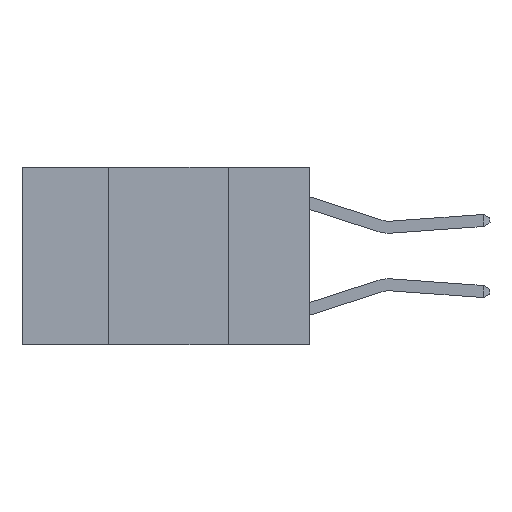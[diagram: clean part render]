
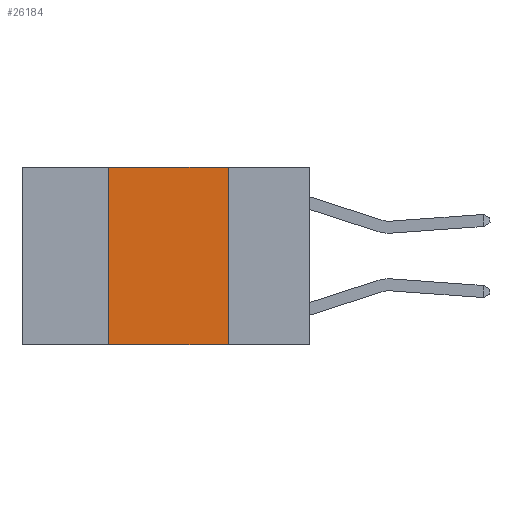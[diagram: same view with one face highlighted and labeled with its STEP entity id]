
A CAD part, left-side view. The second image highlights one B-rep face of the part: STEP entity #26184.
In plain terms, the highlighted planar face has unit normal (-1, 0, 0).
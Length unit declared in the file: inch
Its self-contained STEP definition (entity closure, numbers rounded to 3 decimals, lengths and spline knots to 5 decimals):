
#524 = EDGE_CURVE ( 'NONE', #18201, #8079, #8153, .T. ) ;
#2376 = DIRECTION ( 'NONE',  ( 0., -1., 0. ) ) ;
#2555 = CARTESIAN_POINT ( 'NONE',  ( 0., 0.6, 0. ) ) ;
#3395 = ORIENTED_EDGE ( 'NONE', *, *, #8942, .F. ) ;
#3630 = DIRECTION ( 'NONE',  ( 0., 0., -1. ) ) ;
#4946 = DIRECTION ( 'NONE',  ( 0., 0., -1. ) ) ;
#5600 = VERTEX_POINT ( 'NONE', #19260 ) ;
#8079 = VERTEX_POINT ( 'NONE', #11040 ) ;
#8153 = LINE ( 'NONE', #20246, #26360 ) ;
#8942 = EDGE_CURVE ( 'NONE', #18201, #5600, #16003, .T. ) ;
#9214 = CARTESIAN_POINT ( 'NONE',  ( 0., 0.42, 0. ) ) ;
#9256 = ORIENTED_EDGE ( 'NONE', *, *, #22023, .F. ) ;
#9957 = CARTESIAN_POINT ( 'NONE',  ( 0., 0.17, 0. ) ) ;
#10371 = VECTOR ( 'NONE', #13466, 39.37008 ) ;
#10867 = EDGE_LOOP ( 'NONE', ( #17440, #9256, #3395, #15001 ) ) ;
#11040 = CARTESIAN_POINT ( 'NONE',  ( 0., 0.17, -0.37 ) ) ;
#11109 = CARTESIAN_POINT ( 'NONE',  ( 0., 0.6, 0. ) ) ;
#13101 = CARTESIAN_POINT ( 'NONE',  ( 0., 0.42, -0.37 ) ) ;
#13466 = DIRECTION ( 'NONE',  ( 0., -1., 0. ) ) ;
#14382 = PLANE ( 'NONE',  #23465 ) ;
#15001 = ORIENTED_EDGE ( 'NONE', *, *, #524, .T. ) ;
#15953 = LINE ( 'NONE', #11109, #10371 ) ;
#16003 = LINE ( 'NONE', #9214, #20071 ) ;
#17440 = ORIENTED_EDGE ( 'NONE', *, *, #27719, .F. ) ;
#18201 = VERTEX_POINT ( 'NONE', #13101 ) ;
#19166 = DIRECTION ( 'NONE',  ( 1., 0., 0. ) ) ;
#19260 = CARTESIAN_POINT ( 'NONE',  ( 0., 0.42, 0. ) ) ;
#20071 = VECTOR ( 'NONE', #30572, 39.37008 ) ;
#20241 = VERTEX_POINT ( 'NONE', #9957 ) ;
#20246 = CARTESIAN_POINT ( 'NONE',  ( 0., 0.6, -0.37 ) ) ;
#20321 = CARTESIAN_POINT ( 'NONE',  ( 0., 0.17, 0. ) ) ;
#21672 = FACE_OUTER_BOUND ( 'NONE', #10867, .T. ) ;
#22023 = EDGE_CURVE ( 'NONE', #5600, #20241, #15953, .T. ) ;
#23465 = AXIS2_PLACEMENT_3D ( 'NONE', #2555, #19166, #4946 ) ;
#25622 = VECTOR ( 'NONE', #3630, 39.37008 ) ;
#26184 = ADVANCED_FACE ( 'NONE', ( #21672 ), #14382, .F. ) ;
#26360 = VECTOR ( 'NONE', #2376, 39.37008 ) ;
#27109 = LINE ( 'NONE', #20321, #25622 ) ;
#27719 = EDGE_CURVE ( 'NONE', #20241, #8079, #27109, .T. ) ;
#30572 = DIRECTION ( 'NONE',  ( 0., 0., 1. ) ) ;
